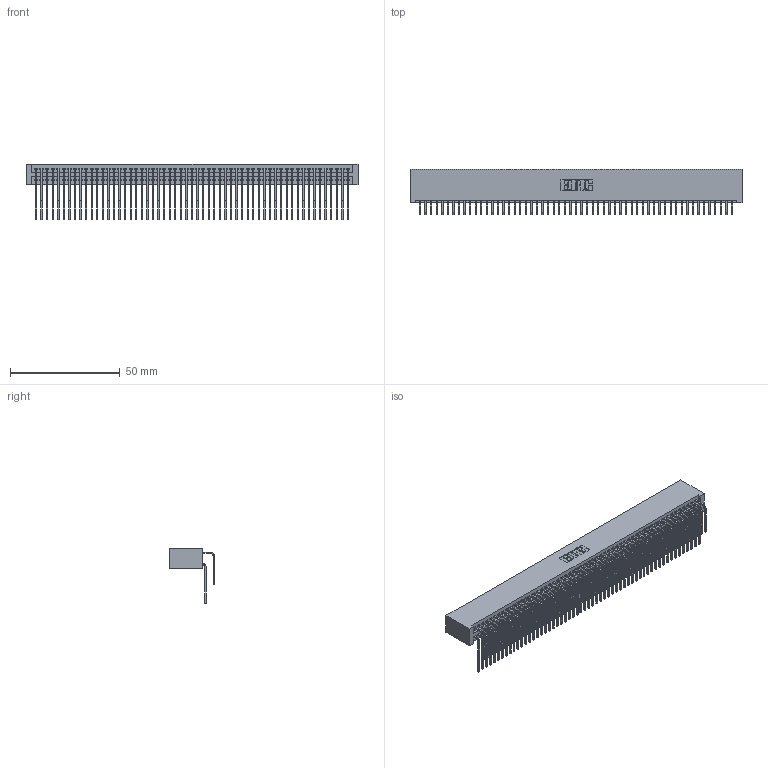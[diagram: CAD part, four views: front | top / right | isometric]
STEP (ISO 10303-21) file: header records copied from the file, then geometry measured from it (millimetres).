
FILE_DESCRIPTION (( 'STEP AP203' ), '1' );
FILE_NAME ('345-114-559-201.STEP', '2019-11-05T12:55:58', ( '' ), ( '' ), 'SwSTEP 2.0', 'SolidWorks 2016', '' );
FILE_SCHEMA (( 'CONFIG_CONTROL_DESIGN' ));
Length unit declared in the file: inch
Products named in the file (4): 345-292-001_558 559 Tail - 1; 345 Part_No Mounting Lugs; 345-114-559-201; 345-292-001_559 Tail - 2
Assembly tree (115 placements, depth 2):
  345-114-559-201
    345 Part_No Mounting Lugs
    345-292-001_558 559 Tail - 1  x57
    345-292-001_559 Tail - 2  x57
Bounding box: 151.38 x 20.56 x 25.53 mm (x, y, z)
Volume: 16118.4 mm3; surface area: 27511.9 mm2
Topology: 115 solids, 115 shells, 6046 faces, 17987 edges, 11838 vertices
Faces by surface type: plane 4066, cylinder 1980
Entity records: 44079 total; most frequent: CARTESIAN_POINT 7419, ORIENTED_EDGE 7302, DIRECTION 6491, EDGE_CURVE 3651, VECTOR 3259, LINE 3259, VERTEX_POINT 2430, AXIS2_PLACEMENT_3D 1616
